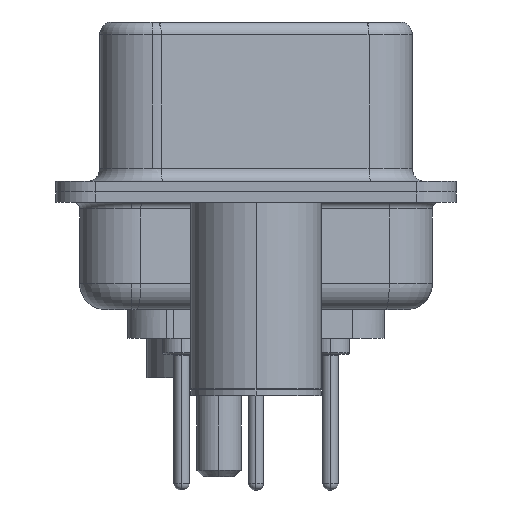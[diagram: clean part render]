
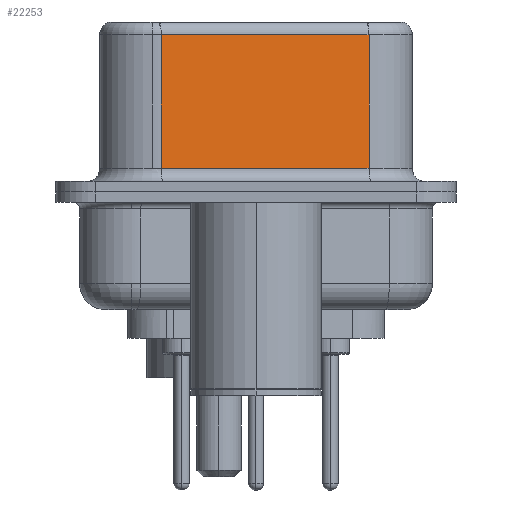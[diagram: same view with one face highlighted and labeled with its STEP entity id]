
A CAD part, left-side view. The second image highlights one B-rep face of the part: STEP entity #22253.
In plain terms, the highlighted planar face has unit normal (-0.985, -0.174, 0).
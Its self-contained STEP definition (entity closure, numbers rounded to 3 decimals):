
#3327 = VERTEX_POINT ( 'NONE', #11090 ) ;
#4014 = EDGE_CURVE ( 'NONE', #29124, #3327, #5940, .T. ) ;
#4175 = CARTESIAN_POINT ( 'NONE',  ( 3.73, 3.628, 0.9 ) ) ;
#4368 = CARTESIAN_POINT ( 'NONE',  ( 3.73, 3.628, 6.52 ) ) ;
#5761 = VECTOR ( 'NONE', #30622, 1000. ) ;
#5940 = LINE ( 'NONE', #14404, #27577 ) ;
#7087 = LINE ( 'NONE', #11846, #7463 ) ;
#7181 = CARTESIAN_POINT ( 'NONE',  ( 5.132, -4.322, 6.52 ) ) ;
#7388 = LINE ( 'NONE', #4368, #5761 ) ;
#7463 = VECTOR ( 'NONE', #24865, 1000. ) ;
#11090 = CARTESIAN_POINT ( 'NONE',  ( 5.132, -4.322, 0.9 ) ) ;
#11138 = CARTESIAN_POINT ( 'NONE',  ( 5.132, -4.322, 6.02 ) ) ;
#11846 = CARTESIAN_POINT ( 'NONE',  ( 5.132, -4.322, 6.02 ) ) ;
#11974 = DIRECTION ( 'NONE',  ( 0., 0., -1. ) ) ;
#12057 = FACE_OUTER_BOUND ( 'NONE', #25731, .T. ) ;
#12372 = PLANE ( 'NONE',  #16592 ) ;
#12421 = VECTOR ( 'NONE', #11974, 1000. ) ;
#12925 = ORIENTED_EDGE ( 'NONE', *, *, #14306, .F. ) ;
#13300 = ORIENTED_EDGE ( 'NONE', *, *, #16616, .T. ) ;
#13667 = ORIENTED_EDGE ( 'NONE', *, *, #26725, .T. ) ;
#14306 = EDGE_CURVE ( 'NONE', #31698, #3327, #18204, .T. ) ;
#14404 = CARTESIAN_POINT ( 'NONE',  ( 5.132, -4.322, 0.9 ) ) ;
#14578 = ORIENTED_EDGE ( 'NONE', *, *, #4014, .T. ) ;
#14879 = DIRECTION ( 'NONE',  ( -0.174, 0.985, 0. ) ) ;
#16592 = AXIS2_PLACEMENT_3D ( 'NONE', #7181, #33011, #14879 ) ;
#16616 = EDGE_CURVE ( 'NONE', #31698, #26538, #7087, .T. ) ;
#18204 = LINE ( 'NONE', #24997, #12421 ) ;
#22253 = ADVANCED_FACE ( 'NONE', ( #12057 ), #12372, .F. ) ;
#22519 = DIRECTION ( 'NONE',  ( 0.174, -0.985, 0. ) ) ;
#24865 = DIRECTION ( 'NONE',  ( -0.174, 0.985, 0. ) ) ;
#24997 = CARTESIAN_POINT ( 'NONE',  ( 5.132, -4.322, 6.52 ) ) ;
#25731 = EDGE_LOOP ( 'NONE', ( #12925, #13300, #13667, #14578 ) ) ;
#26538 = VERTEX_POINT ( 'NONE', #27451 ) ;
#26725 = EDGE_CURVE ( 'NONE', #26538, #29124, #7388, .T. ) ;
#27451 = CARTESIAN_POINT ( 'NONE',  ( 3.73, 3.628, 6.02 ) ) ;
#27577 = VECTOR ( 'NONE', #22519, 1000. ) ;
#29124 = VERTEX_POINT ( 'NONE', #4175 ) ;
#30622 = DIRECTION ( 'NONE',  ( 0., 0., -1. ) ) ;
#31698 = VERTEX_POINT ( 'NONE', #11138 ) ;
#33011 = DIRECTION ( 'NONE',  ( 0.985, 0.174, 0. ) ) ;
